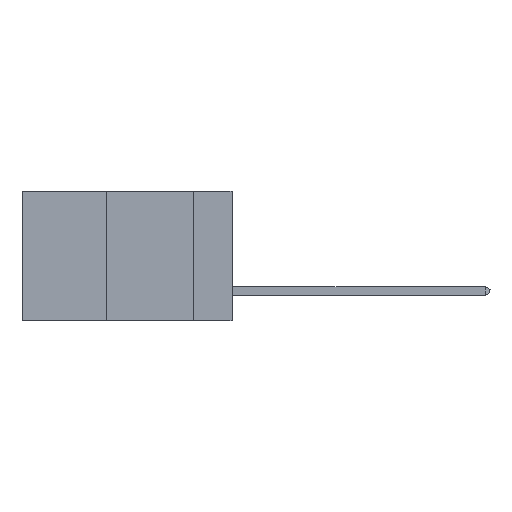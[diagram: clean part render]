
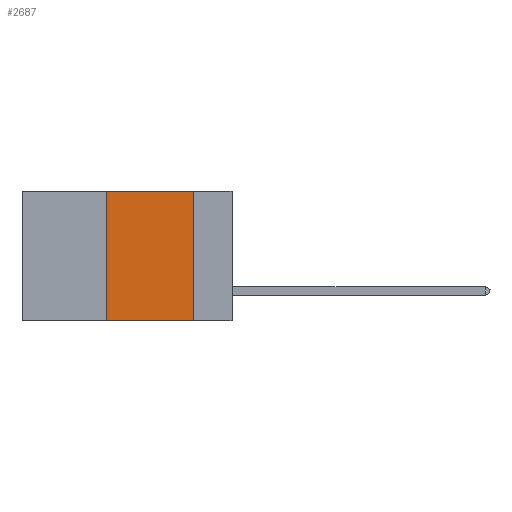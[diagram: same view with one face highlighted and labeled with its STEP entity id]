
A CAD part, left-side view. The second image highlights one B-rep face of the part: STEP entity #2687.
In plain terms, the highlighted planar face has unit normal (-1, 0, 0).
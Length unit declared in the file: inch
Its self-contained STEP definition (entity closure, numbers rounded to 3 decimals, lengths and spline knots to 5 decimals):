
#796 = CARTESIAN_POINT ( 'NONE',  ( 0., 0.6, 0. ) ) ;
#1642 = CARTESIAN_POINT ( 'NONE',  ( 0., 0.36, 0. ) ) ;
#2687 = ADVANCED_FACE ( 'NONE', ( #13659 ), #9699, .F. ) ;
#2947 = CARTESIAN_POINT ( 'NONE',  ( 0., 0.6, 0. ) ) ;
#3148 = DIRECTION ( 'NONE',  ( 0., 0., -1. ) ) ;
#3534 = LINE ( 'NONE', #14696, #27762 ) ;
#3636 = LINE ( 'NONE', #2947, #19464 ) ;
#6491 = CARTESIAN_POINT ( 'NONE',  ( 0., 0.11, 0. ) ) ;
#6779 = EDGE_CURVE ( 'NONE', #24527, #12415, #3534, .T. ) ;
#7611 = EDGE_CURVE ( 'NONE', #27741, #16673, #25986, .T. ) ;
#8263 = DIRECTION ( 'NONE',  ( 0., 0., 1. ) ) ;
#9699 = PLANE ( 'NONE',  #12699 ) ;
#9843 = LINE ( 'NONE', #22270, #11248 ) ;
#11248 = VECTOR ( 'NONE', #15718, 39.37008 ) ;
#12415 = VERTEX_POINT ( 'NONE', #26275 ) ;
#12699 = AXIS2_PLACEMENT_3D ( 'NONE', #796, #27886, #3148 ) ;
#13659 = FACE_OUTER_BOUND ( 'NONE', #28471, .T. ) ;
#14696 = CARTESIAN_POINT ( 'NONE',  ( 0., 0.11, 0. ) ) ;
#15718 = DIRECTION ( 'NONE',  ( 0., -1., 0. ) ) ;
#16673 = VERTEX_POINT ( 'NONE', #18710 ) ;
#17285 = CARTESIAN_POINT ( 'NONE',  ( 0., 0.36, -0.37 ) ) ;
#18672 = DIRECTION ( 'NONE',  ( 0., -1., 0. ) ) ;
#18710 = CARTESIAN_POINT ( 'NONE',  ( 0., 0.36, 0. ) ) ;
#19372 = DIRECTION ( 'NONE',  ( 0., 0., -1. ) ) ;
#19423 = ORIENTED_EDGE ( 'NONE', *, *, #6779, .F. ) ;
#19464 = VECTOR ( 'NONE', #18672, 39.37008 ) ;
#19923 = EDGE_CURVE ( 'NONE', #27741, #12415, #9843, .T. ) ;
#20020 = VECTOR ( 'NONE', #8263, 39.37008 ) ;
#22270 = CARTESIAN_POINT ( 'NONE',  ( 0., 0.6, -0.37 ) ) ;
#22522 = ORIENTED_EDGE ( 'NONE', *, *, #7611, .F. ) ;
#24013 = ORIENTED_EDGE ( 'NONE', *, *, #26957, .F. ) ;
#24527 = VERTEX_POINT ( 'NONE', #6491 ) ;
#25476 = ORIENTED_EDGE ( 'NONE', *, *, #19923, .T. ) ;
#25986 = LINE ( 'NONE', #1642, #20020 ) ;
#26275 = CARTESIAN_POINT ( 'NONE',  ( 0., 0.11, -0.37 ) ) ;
#26957 = EDGE_CURVE ( 'NONE', #16673, #24527, #3636, .T. ) ;
#27741 = VERTEX_POINT ( 'NONE', #17285 ) ;
#27762 = VECTOR ( 'NONE', #19372, 39.37008 ) ;
#27886 = DIRECTION ( 'NONE',  ( 1., 0., 0. ) ) ;
#28471 = EDGE_LOOP ( 'NONE', ( #19423, #24013, #22522, #25476 ) ) ;
